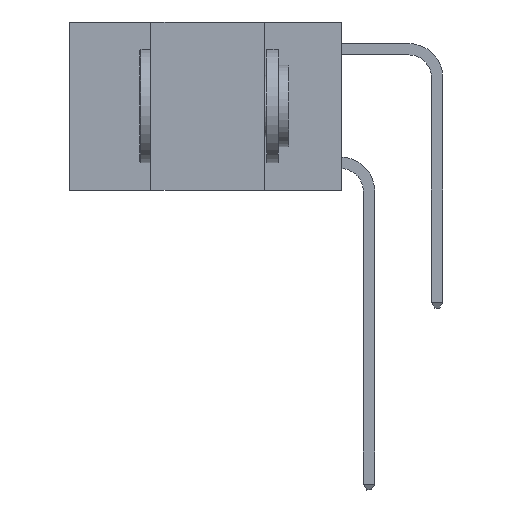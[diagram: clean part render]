
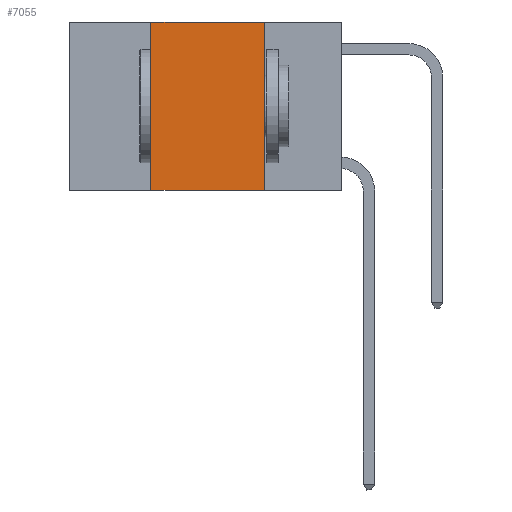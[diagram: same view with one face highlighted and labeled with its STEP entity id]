
A CAD part, left-side view. The second image highlights one B-rep face of the part: STEP entity #7055.
In plain terms, the highlighted planar face has unit normal (-1, 0, 0).
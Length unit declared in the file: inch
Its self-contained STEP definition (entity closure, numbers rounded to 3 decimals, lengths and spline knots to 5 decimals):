
#39 = VECTOR ( 'NONE', #4030, 39.37008 ) ;
#123 = EDGE_CURVE ( 'NONE', #3944, #286, #9285, .T. ) ;
#286 = VERTEX_POINT ( 'NONE', #9561 ) ;
#692 = LINE ( 'NONE', #3968, #39 ) ;
#1030 = PLANE ( 'NONE',  #6390 ) ;
#1240 = ORIENTED_EDGE ( 'NONE', *, *, #8790, .T. ) ;
#1322 = VECTOR ( 'NONE', #5288, 39.37008 ) ;
#1339 = ORIENTED_EDGE ( 'NONE', *, *, #1503, .F. ) ;
#1503 = EDGE_CURVE ( 'NONE', #2097, #11241, #1643, .T. ) ;
#1572 = ORIENTED_EDGE ( 'NONE', *, *, #123, .F. ) ;
#1643 = LINE ( 'NONE', #6766, #10550 ) ;
#1958 = VECTOR ( 'NONE', #9573, 39.37008 ) ;
#2018 = DIRECTION ( 'NONE',  ( 1., 0., 0. ) ) ;
#2097 = VERTEX_POINT ( 'NONE', #6180 ) ;
#2170 = ORIENTED_EDGE ( 'NONE', *, *, #3380, .F. ) ;
#2917 = CARTESIAN_POINT ( 'NONE',  ( 0., 0.6, -0.37 ) ) ;
#3380 = EDGE_CURVE ( 'NONE', #11241, #3944, #692, .T. ) ;
#3944 = VERTEX_POINT ( 'NONE', #11167 ) ;
#3968 = CARTESIAN_POINT ( 'NONE',  ( 0., 0.6, 0. ) ) ;
#4030 = DIRECTION ( 'NONE',  ( 0., -1., 0. ) ) ;
#5288 = DIRECTION ( 'NONE',  ( 0., 0., -1. ) ) ;
#5708 = FACE_OUTER_BOUND ( 'NONE', #8622, .T. ) ;
#6180 = CARTESIAN_POINT ( 'NONE',  ( 0., 0.42, -0.37 ) ) ;
#6390 = AXIS2_PLACEMENT_3D ( 'NONE', #7803, #2018, #8729 ) ;
#6673 = DIRECTION ( 'NONE',  ( 0., 0., 1. ) ) ;
#6766 = CARTESIAN_POINT ( 'NONE',  ( 0., 0.42, 0. ) ) ;
#7055 = ADVANCED_FACE ( 'NONE', ( #5708 ), #1030, .F. ) ;
#7803 = CARTESIAN_POINT ( 'NONE',  ( 0., 0.6, 0. ) ) ;
#8622 = EDGE_LOOP ( 'NONE', ( #1572, #2170, #1339, #1240 ) ) ;
#8729 = DIRECTION ( 'NONE',  ( 0., 0., -1. ) ) ;
#8790 = EDGE_CURVE ( 'NONE', #2097, #286, #11644, .T. ) ;
#9093 = CARTESIAN_POINT ( 'NONE',  ( 0., 0.17, 0. ) ) ;
#9285 = LINE ( 'NONE', #9093, #1322 ) ;
#9561 = CARTESIAN_POINT ( 'NONE',  ( 0., 0.17, -0.37 ) ) ;
#9573 = DIRECTION ( 'NONE',  ( 0., -1., 0. ) ) ;
#9721 = CARTESIAN_POINT ( 'NONE',  ( 0., 0.42, 0. ) ) ;
#10550 = VECTOR ( 'NONE', #6673, 39.37008 ) ;
#11167 = CARTESIAN_POINT ( 'NONE',  ( 0., 0.17, 0. ) ) ;
#11241 = VERTEX_POINT ( 'NONE', #9721 ) ;
#11644 = LINE ( 'NONE', #2917, #1958 ) ;
